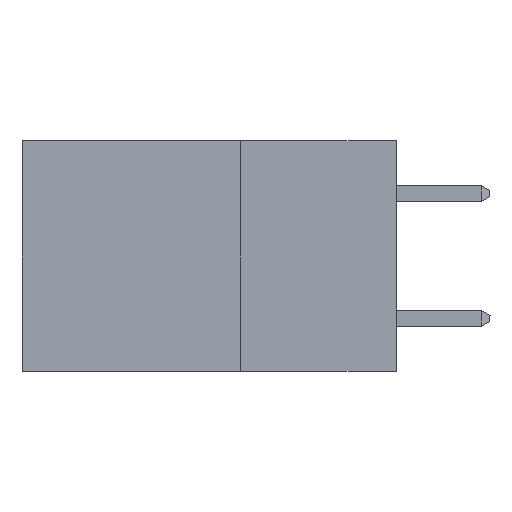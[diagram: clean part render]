
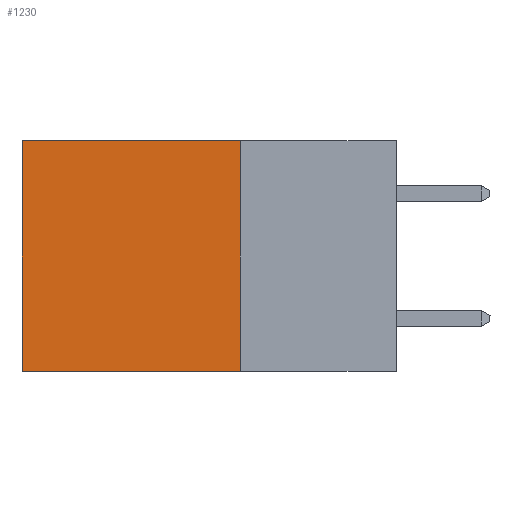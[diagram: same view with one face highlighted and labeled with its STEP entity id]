
A CAD part, left-side view. The second image highlights one B-rep face of the part: STEP entity #1230.
In plain terms, the highlighted planar face has unit normal (-1, 0, 0).
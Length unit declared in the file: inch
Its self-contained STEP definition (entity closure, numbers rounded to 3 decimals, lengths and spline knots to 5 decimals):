
#702 = CARTESIAN_POINT ( 'NONE',  ( 0.2615, 0.25, -0.37 ) ) ;
#1230 = ADVANCED_FACE ( 'NONE', ( #15185 ), #6090, .F. ) ;
#1245 = CARTESIAN_POINT ( 'NONE',  ( 0.2615, 0.25, -0.37 ) ) ;
#1292 = VERTEX_POINT ( 'NONE', #702 ) ;
#1490 = VECTOR ( 'NONE', #19369, 39.37008 ) ;
#2869 = DIRECTION ( 'NONE',  ( 0., 0., -1. ) ) ;
#2948 = DIRECTION ( 'NONE',  ( 1., 0., 0. ) ) ;
#3130 = CARTESIAN_POINT ( 'NONE',  ( 0.2615, 0.25, 0. ) ) ;
#3510 = VECTOR ( 'NONE', #18377, 39.37008 ) ;
#3719 = VERTEX_POINT ( 'NONE', #14689 ) ;
#3973 = CARTESIAN_POINT ( 'NONE',  ( 0.2615, 0.25, -0.37 ) ) ;
#4949 = ORIENTED_EDGE ( 'NONE', *, *, #19941, .F. ) ;
#5857 = CARTESIAN_POINT ( 'NONE',  ( 0.2615, 0.6, 0. ) ) ;
#6090 = PLANE ( 'NONE',  #18615 ) ;
#8232 = VECTOR ( 'NONE', #13977, 39.37008 ) ;
#8426 = LINE ( 'NONE', #1245, #8946 ) ;
#8946 = VECTOR ( 'NONE', #11484, 39.37008 ) ;
#9590 = CARTESIAN_POINT ( 'NONE',  ( 0.2615, 0.25, 0. ) ) ;
#10570 = LINE ( 'NONE', #17688, #1490 ) ;
#11484 = DIRECTION ( 'NONE',  ( 0., 0., -1. ) ) ;
#12327 = VERTEX_POINT ( 'NONE', #5857 ) ;
#12437 = VERTEX_POINT ( 'NONE', #9590 ) ;
#12580 = LINE ( 'NONE', #3130, #3510 ) ;
#13977 = DIRECTION ( 'NONE',  ( 0., 0., -1. ) ) ;
#14458 = ORIENTED_EDGE ( 'NONE', *, *, #21424, .T. ) ;
#14689 = CARTESIAN_POINT ( 'NONE',  ( 0.2615, 0.6, -0.37 ) ) ;
#15185 = FACE_OUTER_BOUND ( 'NONE', #20059, .T. ) ;
#15204 = ORIENTED_EDGE ( 'NONE', *, *, #16722, .T. ) ;
#16722 = EDGE_CURVE ( 'NONE', #12327, #3719, #21652, .T. ) ;
#17688 = CARTESIAN_POINT ( 'NONE',  ( 0.2615, 0.25, -0.37 ) ) ;
#18267 = EDGE_CURVE ( 'NONE', #1292, #3719, #10570, .T. ) ;
#18377 = DIRECTION ( 'NONE',  ( 0., 1., 0. ) ) ;
#18615 = AXIS2_PLACEMENT_3D ( 'NONE', #3973, #2948, #2869 ) ;
#18999 = CARTESIAN_POINT ( 'NONE',  ( 0.2615, 0.6, -0.37 ) ) ;
#19369 = DIRECTION ( 'NONE',  ( 0., 1., 0. ) ) ;
#19941 = EDGE_CURVE ( 'NONE', #12437, #1292, #8426, .T. ) ;
#20059 = EDGE_LOOP ( 'NONE', ( #15204, #20962, #4949, #14458 ) ) ;
#20962 = ORIENTED_EDGE ( 'NONE', *, *, #18267, .F. ) ;
#21424 = EDGE_CURVE ( 'NONE', #12437, #12327, #12580, .T. ) ;
#21652 = LINE ( 'NONE', #18999, #8232 ) ;
